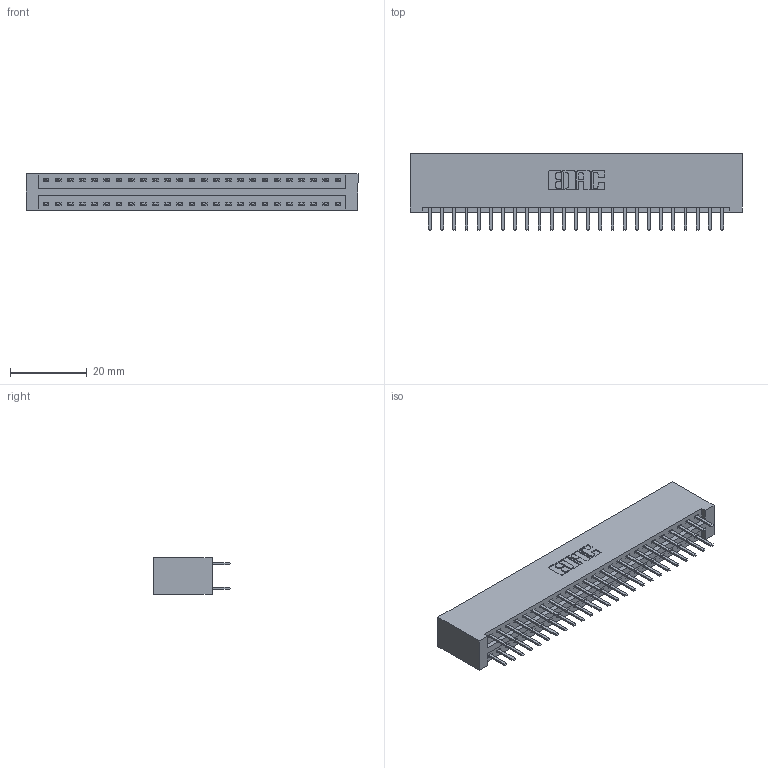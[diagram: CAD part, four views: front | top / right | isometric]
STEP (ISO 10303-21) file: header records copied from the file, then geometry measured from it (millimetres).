
FILE_DESCRIPTION (( 'STEP AP203' ), '1' );
FILE_NAME ('396-050-520-201.STEP', '2018-09-08T02:47:05', ( '' ), ( '' ), 'SwSTEP 2.0', 'SolidWorks 2016', '' );
FILE_SCHEMA (( 'CONFIG_CONTROL_DESIGN' ));
Length unit declared in the file: inch
Products named in the file (3): 346 Part_No Mounting Lugs; 345-292-001_345-293-120; 396-050-520-201
Assembly tree (51 placements, depth 2):
  396-050-520-201
    346 Part_No Mounting Lugs
    345-292-001_345-293-120  x50
Bounding box: 86.61 x 20.02 x 9.4 mm (x, y, z)
Volume: 8865.2 mm3; surface area: 12030.3 mm2
Topology: 51 solids, 51 shells, 2914 faces, 8455 edges, 5502 vertices
Faces by surface type: plane 1922, cylinder 992
Entity records: 18441 total; most frequent: CARTESIAN_POINT 3072, ORIENTED_EDGE 2994, DIRECTION 2741, EDGE_CURVE 1497, VECTOR 1269, LINE 1269, VERTEX_POINT 994, AXIS2_PLACEMENT_3D 736
